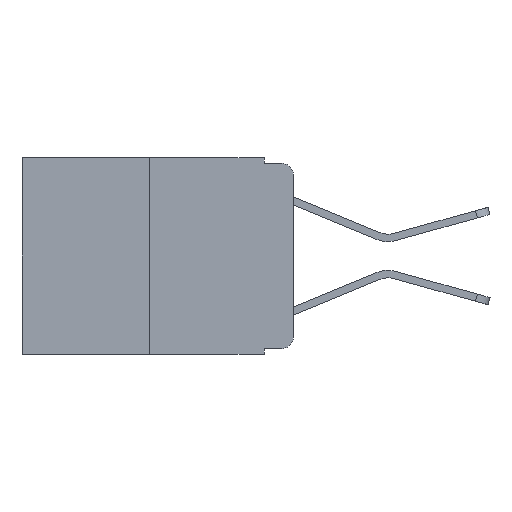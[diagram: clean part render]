
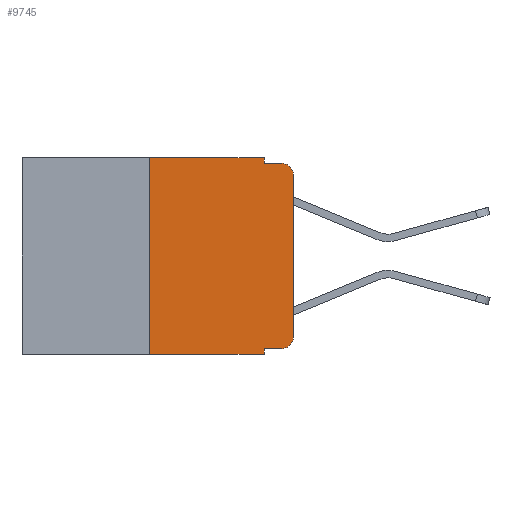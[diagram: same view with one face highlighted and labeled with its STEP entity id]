
A CAD part, left-side view. The second image highlights one B-rep face of the part: STEP entity #9745.
In plain terms, the highlighted planar face has unit normal (-1, 0, 0).
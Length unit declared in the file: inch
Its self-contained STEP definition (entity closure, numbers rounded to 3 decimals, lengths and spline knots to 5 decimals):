
#26 = DIRECTION ( 'NONE',  ( 0., 0., -1. ) ) ;
#51 = DIRECTION ( 'NONE',  ( 1., 0., 0. ) ) ;
#99 = VERTEX_POINT ( 'NONE', #10654 ) ;
#135 = VERTEX_POINT ( 'NONE', #17758 ) ;
#517 = LINE ( 'NONE', #4487, #16687 ) ;
#1847 = CIRCLE ( 'NONE', #13529, 0.02 ) ;
#1932 = DIRECTION ( 'NONE',  ( 0., 0., 1. ) ) ;
#2239 = CARTESIAN_POINT ( 'NONE',  ( 0., 0.25, 0. ) ) ;
#2423 = LINE ( 'NONE', #4911, #6104 ) ;
#2786 = ORIENTED_EDGE ( 'NONE', *, *, #9982, .F. ) ;
#3440 = VECTOR ( 'NONE', #26, 39.37008 ) ;
#3533 = DIRECTION ( 'NONE',  ( 0., 0., -1. ) ) ;
#4220 = EDGE_LOOP ( 'NONE', ( #9780, #14807, #5443, #5754, #2786, #18073, #16280, #6721, #4305, #7014 ) ) ;
#4305 = ORIENTED_EDGE ( 'NONE', *, *, #9807, .T. ) ;
#4317 = CARTESIAN_POINT ( 'NONE',  ( 0., 0.051, -0.01 ) ) ;
#4487 = CARTESIAN_POINT ( 'NONE',  ( 0., 0.051, -0.333 ) ) ;
#4911 = CARTESIAN_POINT ( 'NONE',  ( 0., 0., 0. ) ) ;
#4975 = DIRECTION ( 'NONE',  ( 0., 0., 1. ) ) ;
#5263 = LINE ( 'NONE', #4317, #7455 ) ;
#5312 = CARTESIAN_POINT ( 'NONE',  ( 0., 0.02, -0.03 ) ) ;
#5443 = ORIENTED_EDGE ( 'NONE', *, *, #19569, .F. ) ;
#5754 = ORIENTED_EDGE ( 'NONE', *, *, #12182, .F. ) ;
#6039 = VERTEX_POINT ( 'NONE', #11775 ) ;
#6104 = VECTOR ( 'NONE', #4975, 39.37008 ) ;
#6721 = ORIENTED_EDGE ( 'NONE', *, *, #11764, .F. ) ;
#6757 = DIRECTION ( 'NONE',  ( 0., -1., 0. ) ) ;
#7014 = ORIENTED_EDGE ( 'NONE', *, *, #15829, .T. ) ;
#7218 = VERTEX_POINT ( 'NONE', #10504 ) ;
#7378 = VECTOR ( 'NONE', #9683, 39.37008 ) ;
#7455 = VECTOR ( 'NONE', #17228, 39.37008 ) ;
#7894 = CARTESIAN_POINT ( 'NONE',  ( 0., 0.051, 0. ) ) ;
#8270 = VERTEX_POINT ( 'NONE', #15398 ) ;
#8383 = VECTOR ( 'NONE', #6757, 39.37008 ) ;
#8627 = DIRECTION ( 'NONE',  ( 0., 0., -1. ) ) ;
#8652 = EDGE_CURVE ( 'NONE', #135, #14808, #11370, .T. ) ;
#8688 = CARTESIAN_POINT ( 'NONE',  ( 0., 0.051, 0. ) ) ;
#8891 = CARTESIAN_POINT ( 'NONE',  ( 0., 0., -0.03 ) ) ;
#9114 = FACE_OUTER_BOUND ( 'NONE', #4220, .T. ) ;
#9198 = CARTESIAN_POINT ( 'NONE',  ( 0., 0.02, -0.313 ) ) ;
#9516 = VERTEX_POINT ( 'NONE', #17990 ) ;
#9683 = DIRECTION ( 'NONE',  ( 0., -1., 0. ) ) ;
#9745 = ADVANCED_FACE ( 'NONE', ( #9114 ), #12506, .F. ) ;
#9780 = ORIENTED_EDGE ( 'NONE', *, *, #13074, .T. ) ;
#9807 = EDGE_CURVE ( 'NONE', #19006, #8270, #517, .T. ) ;
#9982 = EDGE_CURVE ( 'NONE', #14808, #9516, #14982, .T. ) ;
#10504 = CARTESIAN_POINT ( 'NONE',  ( 0., 0.051, -0.01 ) ) ;
#10654 = CARTESIAN_POINT ( 'NONE',  ( 0., 0.02, -0.01 ) ) ;
#10787 = DIRECTION ( 'NONE',  ( 0., 0., -1. ) ) ;
#10884 = CARTESIAN_POINT ( 'NONE',  ( 0., 0.473, 0. ) ) ;
#11370 = LINE ( 'NONE', #20260, #15777 ) ;
#11391 = CIRCLE ( 'NONE', #18108, 0.02 ) ;
#11551 = DIRECTION ( 'NONE',  ( -1., 0., 0. ) ) ;
#11764 = EDGE_CURVE ( 'NONE', #19006, #6039, #11789, .T. ) ;
#11775 = CARTESIAN_POINT ( 'NONE',  ( 0., 0.051, -0.343 ) ) ;
#11789 = LINE ( 'NONE', #7894, #3440 ) ;
#11872 = EDGE_CURVE ( 'NONE', #135, #6039, #19121, .T. ) ;
#12182 = EDGE_CURVE ( 'NONE', #9516, #7218, #19828, .T. ) ;
#12272 = VERTEX_POINT ( 'NONE', #8891 ) ;
#12506 = PLANE ( 'NONE',  #17259 ) ;
#12740 = VECTOR ( 'NONE', #8627, 39.37008 ) ;
#12945 = VERTEX_POINT ( 'NONE', #16809 ) ;
#13074 = EDGE_CURVE ( 'NONE', #12945, #12272, #2423, .T. ) ;
#13529 = AXIS2_PLACEMENT_3D ( 'NONE', #5312, #11551, #3533 ) ;
#13854 = DIRECTION ( 'NONE',  ( 0., 0., -1. ) ) ;
#14807 = ORIENTED_EDGE ( 'NONE', *, *, #19179, .T. ) ;
#14808 = VERTEX_POINT ( 'NONE', #2239 ) ;
#14982 = LINE ( 'NONE', #17962, #8383 ) ;
#15398 = CARTESIAN_POINT ( 'NONE',  ( 0., 0.02, -0.333 ) ) ;
#15777 = VECTOR ( 'NONE', #1932, 39.37008 ) ;
#15829 = EDGE_CURVE ( 'NONE', #8270, #12945, #11391, .T. ) ;
#16280 = ORIENTED_EDGE ( 'NONE', *, *, #11872, .T. ) ;
#16687 = VECTOR ( 'NONE', #20156, 39.37008 ) ;
#16809 = CARTESIAN_POINT ( 'NONE',  ( 0., 0., -0.313 ) ) ;
#17037 = CARTESIAN_POINT ( 'NONE',  ( 0., 0.051, -0.333 ) ) ;
#17228 = DIRECTION ( 'NONE',  ( 0., -1., 0. ) ) ;
#17259 = AXIS2_PLACEMENT_3D ( 'NONE', #10884, #51, #13854 ) ;
#17758 = CARTESIAN_POINT ( 'NONE',  ( 0., 0.25, -0.343 ) ) ;
#17962 = CARTESIAN_POINT ( 'NONE',  ( 0., 0.473, 0. ) ) ;
#17990 = CARTESIAN_POINT ( 'NONE',  ( 0., 0.051, 0. ) ) ;
#18073 = ORIENTED_EDGE ( 'NONE', *, *, #8652, .F. ) ;
#18108 = AXIS2_PLACEMENT_3D ( 'NONE', #9198, #20123, #10787 ) ;
#19006 = VERTEX_POINT ( 'NONE', #17037 ) ;
#19121 = LINE ( 'NONE', #19169, #7378 ) ;
#19169 = CARTESIAN_POINT ( 'NONE',  ( 0., 0.473, -0.343 ) ) ;
#19179 = EDGE_CURVE ( 'NONE', #12272, #99, #1847, .T. ) ;
#19569 = EDGE_CURVE ( 'NONE', #7218, #99, #5263, .T. ) ;
#19828 = LINE ( 'NONE', #8688, #12740 ) ;
#20123 = DIRECTION ( 'NONE',  ( -1., 0., 0. ) ) ;
#20156 = DIRECTION ( 'NONE',  ( 0., -1., 0. ) ) ;
#20260 = CARTESIAN_POINT ( 'NONE',  ( 0., 0.25, 0. ) ) ;
